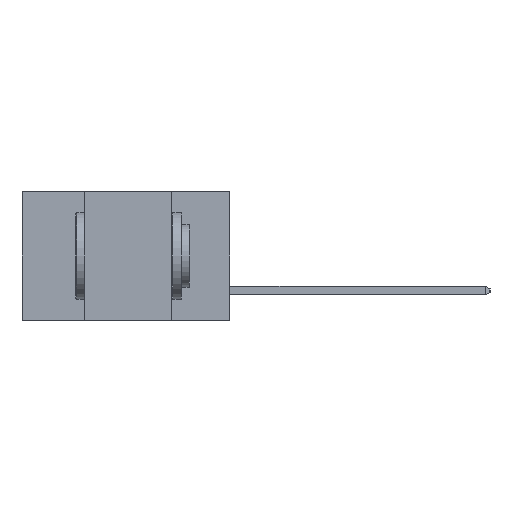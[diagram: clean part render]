
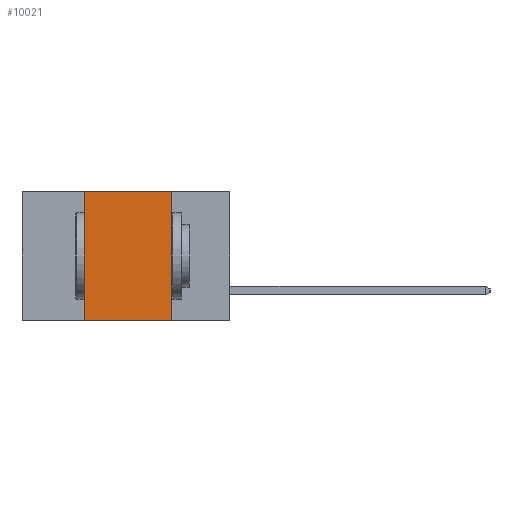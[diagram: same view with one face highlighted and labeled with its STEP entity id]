
A CAD part, left-side view. The second image highlights one B-rep face of the part: STEP entity #10021.
In plain terms, the highlighted planar face has unit normal (-1, 0, 0).
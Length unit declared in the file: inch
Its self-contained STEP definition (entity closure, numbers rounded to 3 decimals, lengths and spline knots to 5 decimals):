
#808 = DIRECTION ( 'NONE',  ( 0., 0., -1. ) ) ;
#1067 = CARTESIAN_POINT ( 'NONE',  ( 0., 0.17, -0.37 ) ) ;
#1248 = LINE ( 'NONE', #5558, #5064 ) ;
#2274 = CARTESIAN_POINT ( 'NONE',  ( 0., 0.6, 0. ) ) ;
#2317 = DIRECTION ( 'NONE',  ( 0., -1., 0. ) ) ;
#5064 = VECTOR ( 'NONE', #13295, 39.37008 ) ;
#5337 = CARTESIAN_POINT ( 'NONE',  ( 0., 0.42, 0. ) ) ;
#5558 = CARTESIAN_POINT ( 'NONE',  ( 0., 0.42, -0.37 ) ) ;
#7117 = VECTOR ( 'NONE', #2317, 39.37008 ) ;
#7137 = EDGE_CURVE ( 'NONE', #17657, #10375, #15765, .T. ) ;
#8153 = EDGE_CURVE ( 'NONE', #10375, #15887, #9243, .T. ) ;
#8867 = ORIENTED_EDGE ( 'NONE', *, *, #17759, .F. ) ;
#9059 = ORIENTED_EDGE ( 'NONE', *, *, #9562, .T. ) ;
#9243 = LINE ( 'NONE', #1067, #12342 ) ;
#9393 = FACE_OUTER_BOUND ( 'NONE', #15895, .T. ) ;
#9562 = EDGE_CURVE ( 'NONE', #14695, #15887, #18001, .T. ) ;
#9646 = DIRECTION ( 'NONE',  ( 0., 0., -1. ) ) ;
#9777 = DIRECTION ( 'NONE',  ( 1., 0., 0. ) ) ;
#9874 = VECTOR ( 'NONE', #15609, 39.37008 ) ;
#10021 = ADVANCED_FACE ( 'NONE', ( #9393 ), #14389, .F. ) ;
#10375 = VERTEX_POINT ( 'NONE', #11266 ) ;
#10584 = AXIS2_PLACEMENT_3D ( 'NONE', #14251, #9777, #9646 ) ;
#11266 = CARTESIAN_POINT ( 'NONE',  ( 0., 0.17, 0. ) ) ;
#12342 = VECTOR ( 'NONE', #808, 39.37008 ) ;
#12936 = ORIENTED_EDGE ( 'NONE', *, *, #7137, .F. ) ;
#13295 = DIRECTION ( 'NONE',  ( 0., 0., 1. ) ) ;
#14251 = CARTESIAN_POINT ( 'NONE',  ( 0., 0.6, 0. ) ) ;
#14389 = PLANE ( 'NONE',  #10584 ) ;
#14695 = VERTEX_POINT ( 'NONE', #19303 ) ;
#15609 = DIRECTION ( 'NONE',  ( 0., -1., 0. ) ) ;
#15652 = CARTESIAN_POINT ( 'NONE',  ( 0., 0.6, -0.37 ) ) ;
#15765 = LINE ( 'NONE', #2274, #7117 ) ;
#15887 = VERTEX_POINT ( 'NONE', #19122 ) ;
#15895 = EDGE_LOOP ( 'NONE', ( #19746, #12936, #8867, #9059 ) ) ;
#17657 = VERTEX_POINT ( 'NONE', #5337 ) ;
#17759 = EDGE_CURVE ( 'NONE', #14695, #17657, #1248, .T. ) ;
#18001 = LINE ( 'NONE', #15652, #9874 ) ;
#19122 = CARTESIAN_POINT ( 'NONE',  ( 0., 0.17, -0.37 ) ) ;
#19303 = CARTESIAN_POINT ( 'NONE',  ( 0., 0.42, -0.37 ) ) ;
#19746 = ORIENTED_EDGE ( 'NONE', *, *, #8153, .F. ) ;
